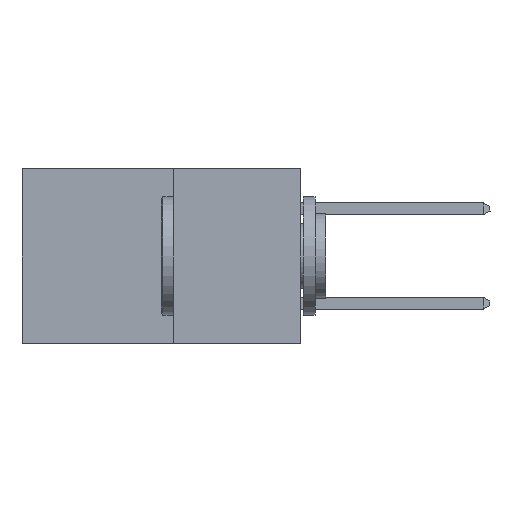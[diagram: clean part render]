
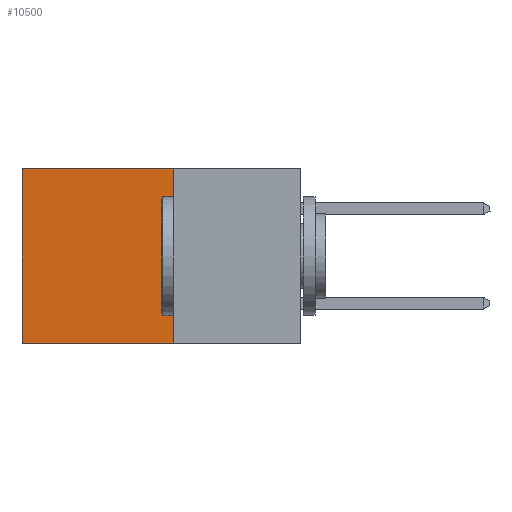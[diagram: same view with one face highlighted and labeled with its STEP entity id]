
A CAD part, left-side view. The second image highlights one B-rep face of the part: STEP entity #10500.
In plain terms, the highlighted planar face has unit normal (-1, 0, 0).
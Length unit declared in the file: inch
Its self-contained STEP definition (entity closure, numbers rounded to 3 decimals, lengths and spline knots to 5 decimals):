
#864 = CARTESIAN_POINT ( 'NONE',  ( 0.277, 0.27, -0.37 ) ) ;
#1944 = CARTESIAN_POINT ( 'NONE',  ( 0.277, 0.27, -0.37 ) ) ;
#2748 = VECTOR ( 'NONE', #9805, 39.37008 ) ;
#3031 = CARTESIAN_POINT ( 'NONE',  ( 0.277, 0.59, -0.37 ) ) ;
#3342 = PLANE ( 'NONE',  #12444 ) ;
#4281 = VECTOR ( 'NONE', #16435, 39.37008 ) ;
#5022 = DIRECTION ( 'NONE',  ( 0., 0., -1. ) ) ;
#5629 = EDGE_CURVE ( 'NONE', #20056, #7409, #18313, .T. ) ;
#6504 = ORIENTED_EDGE ( 'NONE', *, *, #10361, .T. ) ;
#6732 = LINE ( 'NONE', #19934, #2748 ) ;
#7348 = LINE ( 'NONE', #17577, #11360 ) ;
#7409 = VERTEX_POINT ( 'NONE', #13985 ) ;
#7482 = CARTESIAN_POINT ( 'NONE',  ( 0.277, 0.27, 0. ) ) ;
#9124 = DIRECTION ( 'NONE',  ( 0., 0., -1. ) ) ;
#9436 = EDGE_CURVE ( 'NONE', #19156, #20364, #16034, .T. ) ;
#9805 = DIRECTION ( 'NONE',  ( 0., 0., -1. ) ) ;
#10361 = EDGE_CURVE ( 'NONE', #7409, #20364, #6732, .T. ) ;
#10500 = ADVANCED_FACE ( 'NONE', ( #18140 ), #3342, .F. ) ;
#10620 = EDGE_LOOP ( 'NONE', ( #6504, #19340, #15599, #13861 ) ) ;
#11360 = VECTOR ( 'NONE', #9124, 39.37008 ) ;
#12444 = AXIS2_PLACEMENT_3D ( 'NONE', #13464, #15187, #5022 ) ;
#13464 = CARTESIAN_POINT ( 'NONE',  ( 0.277, 0.27, -0.37 ) ) ;
#13861 = ORIENTED_EDGE ( 'NONE', *, *, #5629, .T. ) ;
#13985 = CARTESIAN_POINT ( 'NONE',  ( 0.277, 0.59, 0. ) ) ;
#15187 = DIRECTION ( 'NONE',  ( 1., 0., 0. ) ) ;
#15481 = VECTOR ( 'NONE', #17764, 39.37008 ) ;
#15599 = ORIENTED_EDGE ( 'NONE', *, *, #21315, .F. ) ;
#16034 = LINE ( 'NONE', #864, #15481 ) ;
#16435 = DIRECTION ( 'NONE',  ( 0., 1., 0. ) ) ;
#17577 = CARTESIAN_POINT ( 'NONE',  ( 0.277, 0.27, -0.37 ) ) ;
#17764 = DIRECTION ( 'NONE',  ( 0., 1., 0. ) ) ;
#18140 = FACE_OUTER_BOUND ( 'NONE', #10620, .T. ) ;
#18313 = LINE ( 'NONE', #21497, #4281 ) ;
#19156 = VERTEX_POINT ( 'NONE', #1944 ) ;
#19340 = ORIENTED_EDGE ( 'NONE', *, *, #9436, .F. ) ;
#19934 = CARTESIAN_POINT ( 'NONE',  ( 0.277, 0.59, -0.37 ) ) ;
#20056 = VERTEX_POINT ( 'NONE', #7482 ) ;
#20364 = VERTEX_POINT ( 'NONE', #3031 ) ;
#21315 = EDGE_CURVE ( 'NONE', #20056, #19156, #7348, .T. ) ;
#21497 = CARTESIAN_POINT ( 'NONE',  ( 0.277, 0.27, 0. ) ) ;
